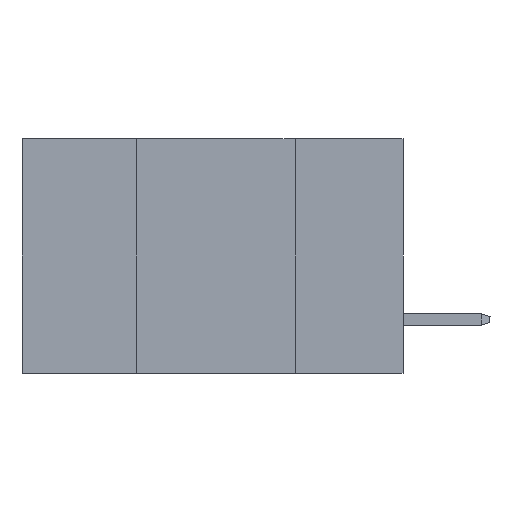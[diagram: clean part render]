
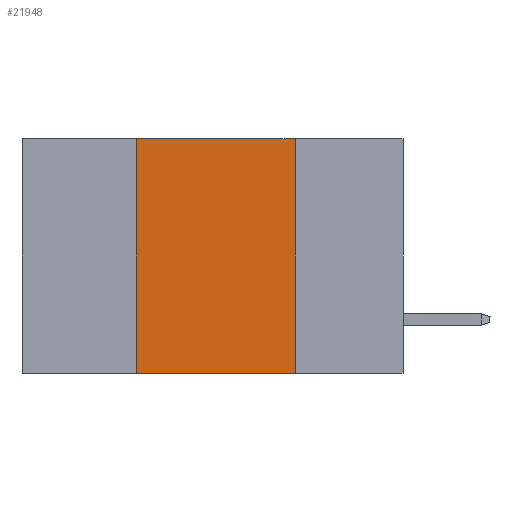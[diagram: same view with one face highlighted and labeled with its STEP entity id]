
A CAD part, left-side view. The second image highlights one B-rep face of the part: STEP entity #21948.
In plain terms, the highlighted planar face has unit normal (-1, 0, 0).
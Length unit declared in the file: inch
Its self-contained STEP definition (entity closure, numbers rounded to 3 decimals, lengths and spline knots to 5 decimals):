
#30 = PLANE ( 'NONE',  #30183 ) ;
#61 = LINE ( 'NONE', #29231, #5987 ) ;
#1422 = VERTEX_POINT ( 'NONE', #24205 ) ;
#1807 = EDGE_CURVE ( 'NONE', #1422, #28970, #17522, .T. ) ;
#2393 = CARTESIAN_POINT ( 'NONE',  ( 0., 0.6, -0.37 ) ) ;
#3955 = ORIENTED_EDGE ( 'NONE', *, *, #11419, .F. ) ;
#4385 = ORIENTED_EDGE ( 'NONE', *, *, #1807, .T. ) ;
#4582 = ORIENTED_EDGE ( 'NONE', *, *, #20301, .F. ) ;
#5135 = CARTESIAN_POINT ( 'NONE',  ( 0., 0.17, 0. ) ) ;
#5987 = VECTOR ( 'NONE', #7131, 39.37008 ) ;
#7131 = DIRECTION ( 'NONE',  ( 0., 0., -1. ) ) ;
#7340 = DIRECTION ( 'NONE',  ( 0., -1., 0. ) ) ;
#7587 = CARTESIAN_POINT ( 'NONE',  ( 0., 0.6, 0. ) ) ;
#8071 = DIRECTION ( 'NONE',  ( 0., -1., 0. ) ) ;
#8651 = VERTEX_POINT ( 'NONE', #5135 ) ;
#11419 = EDGE_CURVE ( 'NONE', #1422, #24607, #28820, .T. ) ;
#12320 = CARTESIAN_POINT ( 'NONE',  ( 0., 0.42, 0. ) ) ;
#17104 = FACE_OUTER_BOUND ( 'NONE', #24581, .T. ) ;
#17209 = ORIENTED_EDGE ( 'NONE', *, *, #26469, .F. ) ;
#17522 = LINE ( 'NONE', #2393, #25405 ) ;
#20301 = EDGE_CURVE ( 'NONE', #8651, #28970, #61, .T. ) ;
#20482 = CARTESIAN_POINT ( 'NONE',  ( 0., 0.6, 0. ) ) ;
#20634 = LINE ( 'NONE', #20482, #24716 ) ;
#21948 = ADVANCED_FACE ( 'NONE', ( #17104 ), #30, .F. ) ;
#24205 = CARTESIAN_POINT ( 'NONE',  ( 0., 0.42, -0.37 ) ) ;
#24581 = EDGE_LOOP ( 'NONE', ( #4582, #17209, #3955, #4385 ) ) ;
#24607 = VERTEX_POINT ( 'NONE', #12320 ) ;
#24716 = VECTOR ( 'NONE', #8071, 39.37008 ) ;
#25405 = VECTOR ( 'NONE', #7340, 39.37008 ) ;
#26326 = CARTESIAN_POINT ( 'NONE',  ( 0., 0.17, -0.37 ) ) ;
#26469 = EDGE_CURVE ( 'NONE', #24607, #8651, #20634, .T. ) ;
#26933 = DIRECTION ( 'NONE',  ( 0., 0., -1. ) ) ;
#28579 = VECTOR ( 'NONE', #31396, 39.37008 ) ;
#28588 = DIRECTION ( 'NONE',  ( 1., 0., 0. ) ) ;
#28820 = LINE ( 'NONE', #29150, #28579 ) ;
#28970 = VERTEX_POINT ( 'NONE', #26326 ) ;
#29150 = CARTESIAN_POINT ( 'NONE',  ( 0., 0.42, 0. ) ) ;
#29231 = CARTESIAN_POINT ( 'NONE',  ( 0., 0.17, 0. ) ) ;
#30183 = AXIS2_PLACEMENT_3D ( 'NONE', #7587, #28588, #26933 ) ;
#31396 = DIRECTION ( 'NONE',  ( 0., 0., 1. ) ) ;
